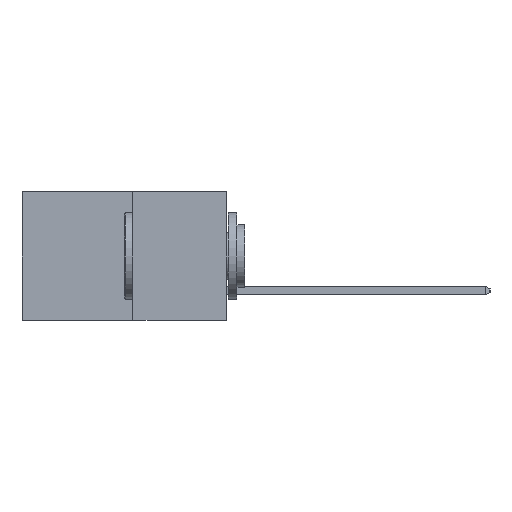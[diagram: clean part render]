
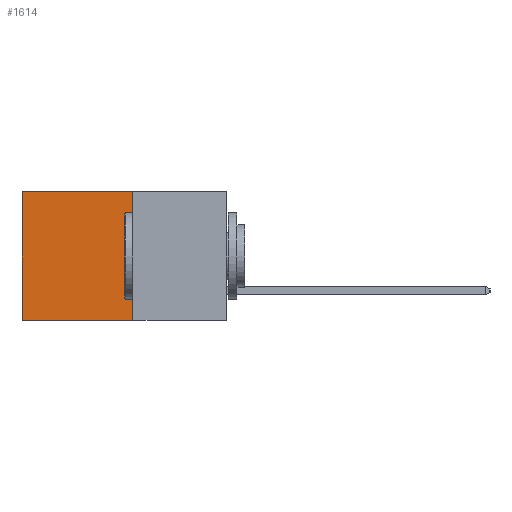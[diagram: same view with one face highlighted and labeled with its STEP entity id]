
A CAD part, left-side view. The second image highlights one B-rep face of the part: STEP entity #1614.
In plain terms, the highlighted planar face has unit normal (-1, 0, 0).
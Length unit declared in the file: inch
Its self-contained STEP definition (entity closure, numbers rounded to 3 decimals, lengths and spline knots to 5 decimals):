
#1269 = EDGE_CURVE ( 'NONE', #7583, #6213, #8744, .T. ) ;
#1614 = ADVANCED_FACE ( 'NONE', ( #9791 ), #5841, .F. ) ;
#2541 = DIRECTION ( 'NONE',  ( 0., 1., 0. ) ) ;
#2725 = LINE ( 'NONE', #10993, #5291 ) ;
#2935 = CARTESIAN_POINT ( 'NONE',  ( 0.277, 0.27, 0. ) ) ;
#3302 = LINE ( 'NONE', #6583, #7348 ) ;
#3454 = ORIENTED_EDGE ( 'NONE', *, *, #3966, .F. ) ;
#3770 = ORIENTED_EDGE ( 'NONE', *, *, #3982, .T. ) ;
#3966 = EDGE_CURVE ( 'NONE', #6213, #6098, #3302, .T. ) ;
#3982 = EDGE_CURVE ( 'NONE', #9742, #6098, #7630, .T. ) ;
#4148 = VECTOR ( 'NONE', #9892, 39.37008 ) ;
#4379 = ORIENTED_EDGE ( 'NONE', *, *, #1269, .F. ) ;
#4511 = DIRECTION ( 'NONE',  ( 0., 0., -1. ) ) ;
#4991 = CARTESIAN_POINT ( 'NONE',  ( 0.277, 0.59, -0.37 ) ) ;
#5291 = VECTOR ( 'NONE', #10213, 39.37008 ) ;
#5295 = EDGE_CURVE ( 'NONE', #7583, #9742, #2725, .T. ) ;
#5450 = ORIENTED_EDGE ( 'NONE', *, *, #5295, .T. ) ;
#5841 = PLANE ( 'NONE',  #8581 ) ;
#5987 = CARTESIAN_POINT ( 'NONE',  ( 0.277, 0.27, -0.37 ) ) ;
#6090 = DIRECTION ( 'NONE',  ( 1., 0., 0. ) ) ;
#6098 = VERTEX_POINT ( 'NONE', #10780 ) ;
#6213 = VERTEX_POINT ( 'NONE', #10347 ) ;
#6215 = DIRECTION ( 'NONE',  ( 0., 0., -1. ) ) ;
#6583 = CARTESIAN_POINT ( 'NONE',  ( 0.277, 0.27, -0.37 ) ) ;
#7089 = VECTOR ( 'NONE', #4511, 39.37008 ) ;
#7348 = VECTOR ( 'NONE', #2541, 39.37008 ) ;
#7583 = VERTEX_POINT ( 'NONE', #2935 ) ;
#7630 = LINE ( 'NONE', #4991, #7089 ) ;
#8581 = AXIS2_PLACEMENT_3D ( 'NONE', #5987, #6090, #6215 ) ;
#8744 = LINE ( 'NONE', #9483, #4148 ) ;
#9060 = CARTESIAN_POINT ( 'NONE',  ( 0.277, 0.59, 0. ) ) ;
#9483 = CARTESIAN_POINT ( 'NONE',  ( 0.277, 0.27, -0.37 ) ) ;
#9742 = VERTEX_POINT ( 'NONE', #9060 ) ;
#9791 = FACE_OUTER_BOUND ( 'NONE', #11088, .T. ) ;
#9892 = DIRECTION ( 'NONE',  ( 0., 0., -1. ) ) ;
#10213 = DIRECTION ( 'NONE',  ( 0., 1., 0. ) ) ;
#10347 = CARTESIAN_POINT ( 'NONE',  ( 0.277, 0.27, -0.37 ) ) ;
#10780 = CARTESIAN_POINT ( 'NONE',  ( 0.277, 0.59, -0.37 ) ) ;
#10993 = CARTESIAN_POINT ( 'NONE',  ( 0.277, 0.27, 0. ) ) ;
#11088 = EDGE_LOOP ( 'NONE', ( #3770, #3454, #4379, #5450 ) ) ;
